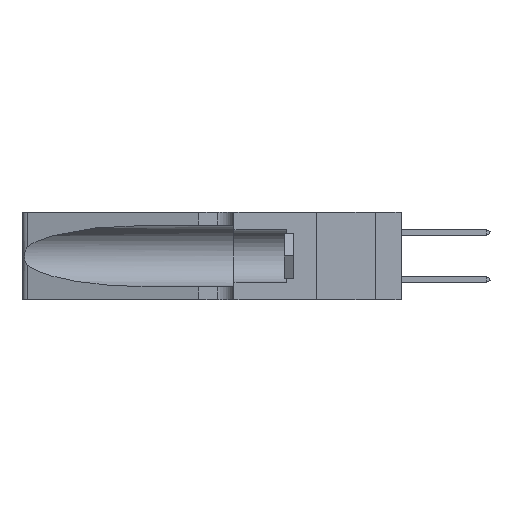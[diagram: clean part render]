
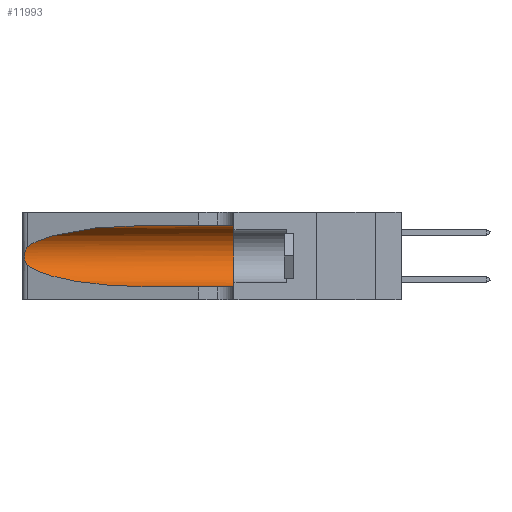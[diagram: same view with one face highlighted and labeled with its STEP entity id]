
A CAD part, left-side view. The second image highlights one B-rep face of the part: STEP entity #11993.
In plain terms, the highlighted cylindrical face has radius 3.308 mm (diameter 6.617 mm), a partial arc.
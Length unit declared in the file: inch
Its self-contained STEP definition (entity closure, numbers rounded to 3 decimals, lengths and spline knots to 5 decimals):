
#976 =( BOUNDED_CURVE ( )  B_SPLINE_CURVE ( 3, ( #40297, #34136, #9039, #12131 ),
 .UNSPECIFIED., .F., .T. ) 
 B_SPLINE_CURVE_WITH_KNOTS ( ( 4, 4 ),
 ( 1.5708, 2.84003 ),
 .UNSPECIFIED. ) 
 CURVE ( )  GEOMETRIC_REPRESENTATION_ITEM ( )  RATIONAL_B_SPLINE_CURVE ( ( 1., 0.87, 0.87, 1. ) ) 
 REPRESENTATION_ITEM ( '' )  );
#1460 = ORIENTED_EDGE ( 'NONE', *, *, #25412, .F. ) ;
#2340 = CARTESIAN_POINT ( 'NONE',  ( 0.26018, 1.23835, 0.19895 ) ) ;
#2868 = CARTESIAN_POINT ( 'NONE',  ( 0.25487, 1.22718, 0.14631 ) ) ;
#3466 = FACE_OUTER_BOUND ( 'NONE', #14011, .T. ) ;
#4475 = CARTESIAN_POINT ( 'NONE',  ( 0.1305, 0.72297, 0.05475 ) ) ;
#4759 = CARTESIAN_POINT ( 'NONE',  ( 0.1305, 1.61858, 0.31525 ) ) ;
#5211 = VERTEX_POINT ( 'NONE', #4475 ) ;
#5741 = EDGE_CURVE ( 'NONE', #6999, #26055, #5816, .T. ) ;
#5816 = B_SPLINE_CURVE_WITH_KNOTS ( 'NONE', 3,
 ( #17208, #10813, #39087, #23471, #24144, #2340, #11876, #36890, #37026, #18411, #18275, #15273, #12138, #2868 ),
 .UNSPECIFIED., .F., .F.,
 ( 4, 2, 2, 2, 2, 2, 4 ),
 ( 0., 0.00027, 0.00053, 0.00107, 0.0016, 0.00187, 0.00214 ),
 .UNSPECIFIED. ) ;
#6126 = ORIENTED_EDGE ( 'NONE', *, *, #19662, .T. ) ;
#6204 = DIRECTION ( 'NONE',  ( 0., 0., -1. ) ) ;
#6999 = VERTEX_POINT ( 'NONE', #23776 ) ;
#7372 = AXIS2_PLACEMENT_3D ( 'NONE', #16932, #22777, #32261 ) ;
#8512 = EDGE_CURVE ( 'NONE', #36967, #34246, #23288, .T. ) ;
#8838 =( BOUNDED_CURVE ( )  B_SPLINE_CURVE ( 3, ( #39875, #14585, #33849, #24258 ),
 .UNSPECIFIED., .F., .T. ) 
 B_SPLINE_CURVE_WITH_KNOTS ( ( 4, 4 ),
 ( 3.44316, 4.71239 ),
 .UNSPECIFIED. ) 
 CURVE ( )  GEOMETRIC_REPRESENTATION_ITEM ( )  RATIONAL_B_SPLINE_CURVE ( ( 1., 0.87, 0.87, 1. ) ) 
 REPRESENTATION_ITEM ( '' )  );
#9039 = CARTESIAN_POINT ( 'NONE',  ( 0.2373, 1.15595, 0.28018 ) ) ;
#10813 = CARTESIAN_POINT ( 'NONE',  ( 0.25555, 1.22994, 0.2215 ) ) ;
#11140 = VECTOR ( 'NONE', #11315, 39.37008 ) ;
#11315 = DIRECTION ( 'NONE',  ( 0., -1., 0. ) ) ;
#11876 = CARTESIAN_POINT ( 'NONE',  ( 0.26075, 1.23896, 0.19203 ) ) ;
#11993 = ADVANCED_FACE ( 'NONE', ( #3466 ), #26899, .F. ) ;
#12131 = CARTESIAN_POINT ( 'NONE',  ( 0.25487, 1.22718, 0.22369 ) ) ;
#12138 = CARTESIAN_POINT ( 'NONE',  ( 0.25555, 1.22993, 0.14849 ) ) ;
#12484 = LINE ( 'NONE', #4759, #15400 ) ;
#12848 = ORIENTED_EDGE ( 'NONE', *, *, #15760, .T. ) ;
#14011 = EDGE_LOOP ( 'NONE', ( #37160, #23594, #6126, #12848, #38721, #1460 ) ) ;
#14585 = CARTESIAN_POINT ( 'NONE',  ( 0.2373, 1.15595, 0.08982 ) ) ;
#15273 = CARTESIAN_POINT ( 'NONE',  ( 0.25639, 1.23186, 0.15144 ) ) ;
#15400 = VECTOR ( 'NONE', #26871, 39.37008 ) ;
#15760 = EDGE_CURVE ( 'NONE', #5211, #34246, #31680, .T. ) ;
#16932 = CARTESIAN_POINT ( 'NONE',  ( 0.1305, 0.35, 0.185 ) ) ;
#17208 = CARTESIAN_POINT ( 'NONE',  ( 0.25487, 1.22718, 0.22369 ) ) ;
#18275 = CARTESIAN_POINT ( 'NONE',  ( 0.25789, 1.23486, 0.15765 ) ) ;
#18411 = CARTESIAN_POINT ( 'NONE',  ( 0.25856, 1.23593, 0.16098 ) ) ;
#18968 = AXIS2_PLACEMENT_3D ( 'NONE', #27306, #23746, #6204 ) ;
#19662 = EDGE_CURVE ( 'NONE', #26055, #5211, #8838, .T. ) ;
#22777 = DIRECTION ( 'NONE',  ( 0., 1., 0. ) ) ;
#23288 = CIRCLE ( 'NONE', #7372, 0.13025 ) ;
#23471 = CARTESIAN_POINT ( 'NONE',  ( 0.25787, 1.23484, 0.2124 ) ) ;
#23594 = ORIENTED_EDGE ( 'NONE', *, *, #5741, .T. ) ;
#23746 = DIRECTION ( 'NONE',  ( 0., -1., 0. ) ) ;
#23776 = CARTESIAN_POINT ( 'NONE',  ( 0.25487, 1.22718, 0.22369 ) ) ;
#24144 = CARTESIAN_POINT ( 'NONE',  ( 0.25854, 1.2359, 0.20912 ) ) ;
#24258 = CARTESIAN_POINT ( 'NONE',  ( 0.1305, 0.72297, 0.05475 ) ) ;
#25412 = EDGE_CURVE ( 'NONE', #37843, #36967, #12484, .T. ) ;
#26055 = VERTEX_POINT ( 'NONE', #32175 ) ;
#26871 = DIRECTION ( 'NONE',  ( 0., -1., 0. ) ) ;
#26887 = CARTESIAN_POINT ( 'NONE',  ( 0.1305, 1.61858, 0.05475 ) ) ;
#26899 = CYLINDRICAL_SURFACE ( 'NONE', #18968, 0.13025 ) ;
#27306 = CARTESIAN_POINT ( 'NONE',  ( 0.1305, 1.61858, 0.185 ) ) ;
#29188 = CARTESIAN_POINT ( 'NONE',  ( 0.1305, 0.35, 0.05475 ) ) ;
#31333 = EDGE_CURVE ( 'NONE', #37843, #6999, #976, .T. ) ;
#31680 = LINE ( 'NONE', #26887, #11140 ) ;
#32175 = CARTESIAN_POINT ( 'NONE',  ( 0.25487, 1.22718, 0.14631 ) ) ;
#32261 = DIRECTION ( 'NONE',  ( 0., 0., 1. ) ) ;
#33849 = CARTESIAN_POINT ( 'NONE',  ( 0.18966, 0.96281, 0.05475 ) ) ;
#34136 = CARTESIAN_POINT ( 'NONE',  ( 0.18966, 0.96281, 0.31525 ) ) ;
#34246 = VERTEX_POINT ( 'NONE', #29188 ) ;
#35607 = CARTESIAN_POINT ( 'NONE',  ( 0.1305, 0.35, 0.31525 ) ) ;
#36890 = CARTESIAN_POINT ( 'NONE',  ( 0.26075, 1.23896, 0.178 ) ) ;
#36967 = VERTEX_POINT ( 'NONE', #35607 ) ;
#37026 = CARTESIAN_POINT ( 'NONE',  ( 0.26017, 1.23833, 0.17102 ) ) ;
#37160 = ORIENTED_EDGE ( 'NONE', *, *, #31333, .T. ) ;
#37843 = VERTEX_POINT ( 'NONE', #40351 ) ;
#38721 = ORIENTED_EDGE ( 'NONE', *, *, #8512, .F. ) ;
#39087 = CARTESIAN_POINT ( 'NONE',  ( 0.25639, 1.23184, 0.21858 ) ) ;
#39875 = CARTESIAN_POINT ( 'NONE',  ( 0.25487, 1.22718, 0.14631 ) ) ;
#40297 = CARTESIAN_POINT ( 'NONE',  ( 0.1305, 0.72297, 0.31525 ) ) ;
#40351 = CARTESIAN_POINT ( 'NONE',  ( 0.1305, 0.72297, 0.31525 ) ) ;
